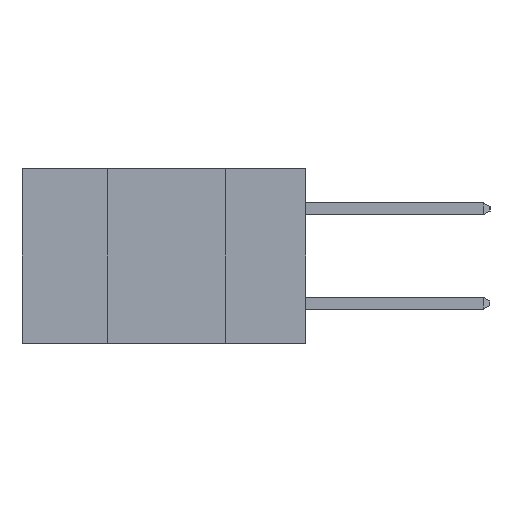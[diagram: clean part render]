
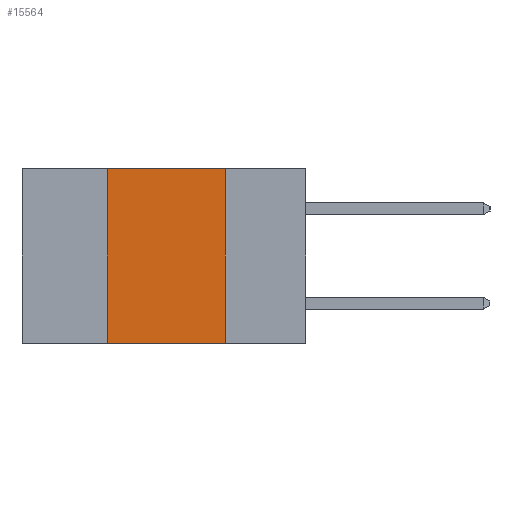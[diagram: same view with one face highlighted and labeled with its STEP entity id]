
A CAD part, left-side view. The second image highlights one B-rep face of the part: STEP entity #15564.
In plain terms, the highlighted planar face has unit normal (-1, 0, 0).
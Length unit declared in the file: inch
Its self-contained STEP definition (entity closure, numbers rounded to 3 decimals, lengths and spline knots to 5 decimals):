
#2452 = EDGE_CURVE ( 'NONE', #17260, #10049, #3081, .T. ) ;
#2573 = CARTESIAN_POINT ( 'NONE',  ( 0., 0.6, 0. ) ) ;
#3081 = LINE ( 'NONE', #3972, #16292 ) ;
#3202 = VERTEX_POINT ( 'NONE', #5763 ) ;
#3972 = CARTESIAN_POINT ( 'NONE',  ( 0., 0.17, 0. ) ) ;
#4742 = EDGE_CURVE ( 'NONE', #8968, #3202, #5728, .T. ) ;
#4999 = CARTESIAN_POINT ( 'NONE',  ( 0., 0.6, -0.37 ) ) ;
#5005 = CARTESIAN_POINT ( 'NONE',  ( 0., 0.42, -0.37 ) ) ;
#5562 = VECTOR ( 'NONE', #18774, 39.37008 ) ;
#5728 = LINE ( 'NONE', #17885, #14339 ) ;
#5763 = CARTESIAN_POINT ( 'NONE',  ( 0., 0.42, 0. ) ) ;
#6020 = CARTESIAN_POINT ( 'NONE',  ( 0., 0.17, -0.37 ) ) ;
#6033 = DIRECTION ( 'NONE',  ( 1., 0., 0. ) ) ;
#6527 = DIRECTION ( 'NONE',  ( 0., -1., 0. ) ) ;
#6887 = ORIENTED_EDGE ( 'NONE', *, *, #8882, .F. ) ;
#8882 = EDGE_CURVE ( 'NONE', #3202, #17260, #15865, .T. ) ;
#8968 = VERTEX_POINT ( 'NONE', #5005 ) ;
#10049 = VERTEX_POINT ( 'NONE', #6020 ) ;
#10616 = DIRECTION ( 'NONE',  ( 0., 0., -1. ) ) ;
#10965 = EDGE_CURVE ( 'NONE', #8968, #10049, #19872, .T. ) ;
#12028 = ORIENTED_EDGE ( 'NONE', *, *, #4742, .F. ) ;
#14339 = VECTOR ( 'NONE', #17687, 39.37008 ) ;
#15087 = CARTESIAN_POINT ( 'NONE',  ( 0., 0.6, 0. ) ) ;
#15564 = ADVANCED_FACE ( 'NONE', ( #19179 ), #19757, .F. ) ;
#15865 = LINE ( 'NONE', #15087, #20459 ) ;
#16292 = VECTOR ( 'NONE', #10616, 39.37008 ) ;
#16576 = ORIENTED_EDGE ( 'NONE', *, *, #10965, .T. ) ;
#17260 = VERTEX_POINT ( 'NONE', #17615 ) ;
#17615 = CARTESIAN_POINT ( 'NONE',  ( 0., 0.17, 0. ) ) ;
#17687 = DIRECTION ( 'NONE',  ( 0., 0., 1. ) ) ;
#17885 = CARTESIAN_POINT ( 'NONE',  ( 0., 0.42, 0. ) ) ;
#18067 = DIRECTION ( 'NONE',  ( 0., 0., -1. ) ) ;
#18774 = DIRECTION ( 'NONE',  ( 0., -1., 0. ) ) ;
#19179 = FACE_OUTER_BOUND ( 'NONE', #20255, .T. ) ;
#19757 = PLANE ( 'NONE',  #19912 ) ;
#19872 = LINE ( 'NONE', #4999, #5562 ) ;
#19912 = AXIS2_PLACEMENT_3D ( 'NONE', #2573, #6033, #18067 ) ;
#20103 = ORIENTED_EDGE ( 'NONE', *, *, #2452, .F. ) ;
#20255 = EDGE_LOOP ( 'NONE', ( #20103, #6887, #12028, #16576 ) ) ;
#20459 = VECTOR ( 'NONE', #6527, 39.37008 ) ;
